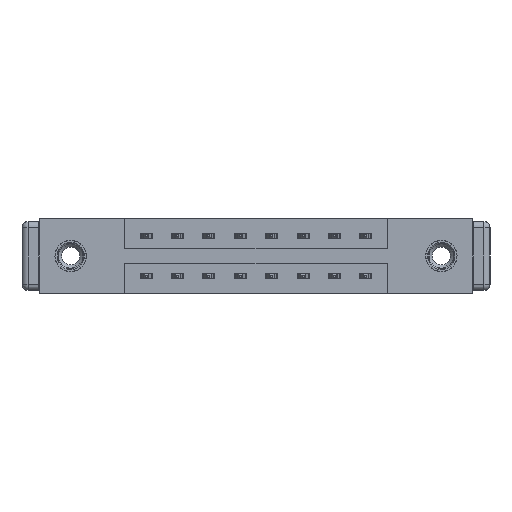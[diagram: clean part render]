
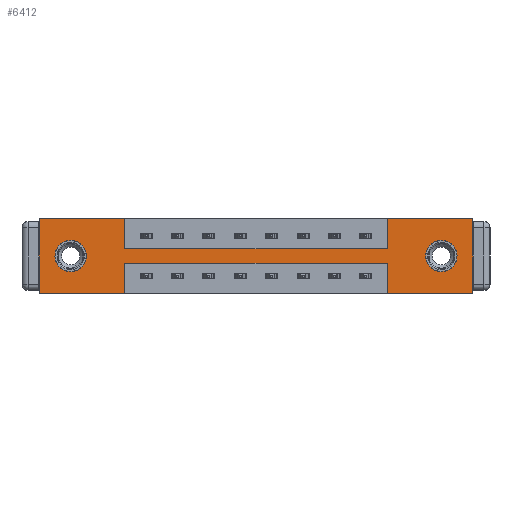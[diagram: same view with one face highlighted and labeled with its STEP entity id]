
A CAD part, front view. The second image highlights one B-rep face of the part: STEP entity #6412.
In plain terms, the highlighted planar face has unit normal (0, -1, 0).
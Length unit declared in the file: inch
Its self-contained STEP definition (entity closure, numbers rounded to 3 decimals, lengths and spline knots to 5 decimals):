
#91 = EDGE_CURVE ( 'NONE', #9414, #9587, #3976, .T. ) ;
#135 = FACE_BOUND ( 'NONE', #7141, .T. ) ;
#146 = VECTOR ( 'NONE', #11348, 39.37008 ) ;
#252 = DIRECTION ( 'NONE',  ( 0., 0., 1. ) ) ;
#331 = ORIENTED_EDGE ( 'NONE', *, *, #1827, .F. ) ;
#419 = DIRECTION ( 'NONE',  ( 0., 1., 0. ) ) ;
#629 = EDGE_CURVE ( 'NONE', #3409, #6597, #10270, .T. ) ;
#816 = ORIENTED_EDGE ( 'NONE', *, *, #9518, .F. ) ;
#857 = CARTESIAN_POINT ( 'NONE',  ( 1.729, 0., -0.15 ) ) ;
#905 = DIRECTION ( 'NONE',  ( 0., 0., -1. ) ) ;
#1058 = VECTOR ( 'NONE', #7113, 39.37008 ) ;
#1096 = CARTESIAN_POINT ( 'NONE',  ( 1.729, 0., -0.22 ) ) ;
#1280 = EDGE_CURVE ( 'NONE', #11914, #5512, #7104, .T. ) ;
#1364 = EDGE_CURVE ( 'NONE', #4600, #7504, #4291, .T. ) ;
#1548 = VECTOR ( 'NONE', #5077, 39.37008 ) ;
#1812 = DIRECTION ( 'NONE',  ( 0., 0., -1. ) ) ;
#1827 = EDGE_CURVE ( 'NONE', #2505, #9414, #9522, .T. ) ;
#1947 = CARTESIAN_POINT ( 'NONE',  ( 0.155, 0., -0.185 ) ) ;
#1994 = DIRECTION ( 'NONE',  ( 0., 0., 1. ) ) ;
#2085 = VERTEX_POINT ( 'NONE', #6038 ) ;
#2135 = LINE ( 'NONE', #4898, #11414 ) ;
#2250 = CARTESIAN_POINT ( 'NONE',  ( 0.155, 0., -0.185 ) ) ;
#2505 = VERTEX_POINT ( 'NONE', #5970 ) ;
#2510 = AXIS2_PLACEMENT_3D ( 'NONE', #1947, #7296, #1994 ) ;
#2540 = ORIENTED_EDGE ( 'NONE', *, *, #8767, .F. ) ;
#2572 = VERTEX_POINT ( 'NONE', #2990 ) ;
#2706 = ORIENTED_EDGE ( 'NONE', *, *, #6896, .F. ) ;
#2822 = PLANE ( 'NONE',  #11782 ) ;
#2990 = CARTESIAN_POINT ( 'NONE',  ( 0.425, 0., -0.22 ) ) ;
#3109 = CARTESIAN_POINT ( 'NONE',  ( 0., 0., 0. ) ) ;
#3409 = VERTEX_POINT ( 'NONE', #11630 ) ;
#3414 = DIRECTION ( 'NONE',  ( 1., 0., 0. ) ) ;
#3439 = CARTESIAN_POINT ( 'NONE',  ( 1.999, 0., -0.185 ) ) ;
#3529 = CARTESIAN_POINT ( 'NONE',  ( 0.425, 0., -0.22 ) ) ;
#3572 = VERTEX_POINT ( 'NONE', #4734 ) ;
#3855 = CARTESIAN_POINT ( 'NONE',  ( 2.154, 0., 0. ) ) ;
#3901 = VECTOR ( 'NONE', #8862, 39.37008 ) ;
#3939 = VERTEX_POINT ( 'NONE', #12723 ) ;
#3976 = LINE ( 'NONE', #6619, #5304 ) ;
#4216 = LINE ( 'NONE', #3529, #12200 ) ;
#4291 = LINE ( 'NONE', #3109, #146 ) ;
#4347 = ORIENTED_EDGE ( 'NONE', *, *, #13234, .F. ) ;
#4410 = ORIENTED_EDGE ( 'NONE', *, *, #8797, .F. ) ;
#4600 = VERTEX_POINT ( 'NONE', #4785 ) ;
#4614 = DIRECTION ( 'NONE',  ( -1., 0., 0. ) ) ;
#4734 = CARTESIAN_POINT ( 'NONE',  ( 1.999, 0., -0.263 ) ) ;
#4779 = EDGE_CURVE ( 'NONE', #8773, #8527, #4991, .T. ) ;
#4784 = CARTESIAN_POINT ( 'NONE',  ( 0.425, 0., 0. ) ) ;
#4785 = CARTESIAN_POINT ( 'NONE',  ( 0., 0., 0. ) ) ;
#4898 = CARTESIAN_POINT ( 'NONE',  ( 0.425, 0., -0.37 ) ) ;
#4899 = LINE ( 'NONE', #6059, #1058 ) ;
#4991 = CIRCLE ( 'NONE', #2510, 0.078 ) ;
#5077 = DIRECTION ( 'NONE',  ( 1., 0., 0. ) ) ;
#5133 = CARTESIAN_POINT ( 'NONE',  ( 1.999, 0., -0.185 ) ) ;
#5273 = FACE_BOUND ( 'NONE', #13248, .T. ) ;
#5304 = VECTOR ( 'NONE', #8513, 39.37008 ) ;
#5512 = VERTEX_POINT ( 'NONE', #6915 ) ;
#5582 = CARTESIAN_POINT ( 'NONE',  ( 0., 0., 0. ) ) ;
#5689 = CARTESIAN_POINT ( 'NONE',  ( 0.425, 0., 0. ) ) ;
#5869 = CIRCLE ( 'NONE', #12159, 0.078 ) ;
#5970 = CARTESIAN_POINT ( 'NONE',  ( 2.154, 0., 0. ) ) ;
#6038 = CARTESIAN_POINT ( 'NONE',  ( 0.425, 0., -0.15 ) ) ;
#6059 = CARTESIAN_POINT ( 'NONE',  ( 0., 0., 0. ) ) ;
#6123 = CARTESIAN_POINT ( 'NONE',  ( 2.154, 0., -0.37 ) ) ;
#6124 = VECTOR ( 'NONE', #12165, 39.37008 ) ;
#6165 = CARTESIAN_POINT ( 'NONE',  ( 0.425, 0., -0.15 ) ) ;
#6405 = AXIS2_PLACEMENT_3D ( 'NONE', #5133, #8371, #8412 ) ;
#6412 = ADVANCED_FACE ( 'NONE', ( #135, #5273, #11950 ), #2822, .T. ) ;
#6597 = VERTEX_POINT ( 'NONE', #13278 ) ;
#6619 = CARTESIAN_POINT ( 'NONE',  ( 0., 0., -0.37 ) ) ;
#6689 = VECTOR ( 'NONE', #7586, 39.37008 ) ;
#6895 = EDGE_CURVE ( 'NONE', #8527, #8773, #7016, .T. ) ;
#6896 = EDGE_CURVE ( 'NONE', #5512, #2505, #10242, .T. ) ;
#6915 = CARTESIAN_POINT ( 'NONE',  ( 1.729, 0., 0. ) ) ;
#6943 = ORIENTED_EDGE ( 'NONE', *, *, #13256, .T. ) ;
#6947 = CARTESIAN_POINT ( 'NONE',  ( 0.155, 0., -0.263 ) ) ;
#7016 = CIRCLE ( 'NONE', #8831, 0.078 ) ;
#7033 = LINE ( 'NONE', #5689, #6689 ) ;
#7104 = LINE ( 'NONE', #11126, #6124 ) ;
#7113 = DIRECTION ( 'NONE',  ( 0., 0., 1. ) ) ;
#7141 = EDGE_LOOP ( 'NONE', ( #12300, #6943 ) ) ;
#7296 = DIRECTION ( 'NONE',  ( 0., 1., 0. ) ) ;
#7504 = VERTEX_POINT ( 'NONE', #4784 ) ;
#7586 = DIRECTION ( 'NONE',  ( 0., 0., -1. ) ) ;
#7851 = CARTESIAN_POINT ( 'NONE',  ( 0., 0., -0.37 ) ) ;
#7904 = EDGE_CURVE ( 'NONE', #3939, #3572, #10973, .T. ) ;
#7933 = DIRECTION ( 'NONE',  ( 0., 0., -1. ) ) ;
#8047 = DIRECTION ( 'NONE',  ( 0., 0., 1. ) ) ;
#8069 = ORIENTED_EDGE ( 'NONE', *, *, #1280, .F. ) ;
#8371 = DIRECTION ( 'NONE',  ( 0., 1., 0. ) ) ;
#8412 = DIRECTION ( 'NONE',  ( 0., 0., -1. ) ) ;
#8513 = DIRECTION ( 'NONE',  ( -1., 0., 0. ) ) ;
#8527 = VERTEX_POINT ( 'NONE', #11638 ) ;
#8681 = CARTESIAN_POINT ( 'NONE',  ( 1.729, 0., -0.37 ) ) ;
#8767 = EDGE_CURVE ( 'NONE', #9587, #9375, #9828, .T. ) ;
#8773 = VERTEX_POINT ( 'NONE', #6947 ) ;
#8797 = EDGE_CURVE ( 'NONE', #2085, #11914, #12739, .T. ) ;
#8831 = AXIS2_PLACEMENT_3D ( 'NONE', #2250, #12695, #252 ) ;
#8862 = DIRECTION ( 'NONE',  ( -1., 0., 0. ) ) ;
#8959 = VECTOR ( 'NONE', #3414, 39.37008 ) ;
#8990 = DIRECTION ( 'NONE',  ( 0., 0., -1. ) ) ;
#9068 = EDGE_LOOP ( 'NONE', ( #11491, #11958, #2540, #9132, #331, #2706, #8069, #4410, #4347, #11704, #816, #9120 ) ) ;
#9120 = ORIENTED_EDGE ( 'NONE', *, *, #629, .F. ) ;
#9132 = ORIENTED_EDGE ( 'NONE', *, *, #91, .F. ) ;
#9375 = VERTEX_POINT ( 'NONE', #1096 ) ;
#9414 = VERTEX_POINT ( 'NONE', #6123 ) ;
#9518 = EDGE_CURVE ( 'NONE', #6597, #4600, #4899, .T. ) ;
#9522 = LINE ( 'NONE', #3855, #12590 ) ;
#9587 = VERTEX_POINT ( 'NONE', #13113 ) ;
#9828 = LINE ( 'NONE', #8681, #9996 ) ;
#9872 = EDGE_CURVE ( 'NONE', #2572, #3409, #2135, .T. ) ;
#9996 = VECTOR ( 'NONE', #8047, 39.37008 ) ;
#10242 = LINE ( 'NONE', #5582, #8959 ) ;
#10270 = LINE ( 'NONE', #7851, #3901 ) ;
#10973 = CIRCLE ( 'NONE', #6405, 0.078 ) ;
#11069 = CARTESIAN_POINT ( 'NONE',  ( 0., 0., -0.37 ) ) ;
#11108 = DIRECTION ( 'NONE',  ( 0., -1., 0. ) ) ;
#11126 = CARTESIAN_POINT ( 'NONE',  ( 1.729, 0., 0. ) ) ;
#11348 = DIRECTION ( 'NONE',  ( 1., 0., 0. ) ) ;
#11414 = VECTOR ( 'NONE', #905, 39.37008 ) ;
#11491 = ORIENTED_EDGE ( 'NONE', *, *, #9872, .F. ) ;
#11630 = CARTESIAN_POINT ( 'NONE',  ( 0.425, 0., -0.37 ) ) ;
#11638 = CARTESIAN_POINT ( 'NONE',  ( 0.155, 0., -0.107 ) ) ;
#11704 = ORIENTED_EDGE ( 'NONE', *, *, #1364, .F. ) ;
#11782 = AXIS2_PLACEMENT_3D ( 'NONE', #11069, #11108, #8990 ) ;
#11914 = VERTEX_POINT ( 'NONE', #857 ) ;
#11950 = FACE_OUTER_BOUND ( 'NONE', #9068, .T. ) ;
#11958 = ORIENTED_EDGE ( 'NONE', *, *, #13231, .F. ) ;
#12159 = AXIS2_PLACEMENT_3D ( 'NONE', #3439, #419, #7933 ) ;
#12165 = DIRECTION ( 'NONE',  ( 0., 0., 1. ) ) ;
#12200 = VECTOR ( 'NONE', #4614, 39.37008 ) ;
#12300 = ORIENTED_EDGE ( 'NONE', *, *, #7904, .T. ) ;
#12590 = VECTOR ( 'NONE', #1812, 39.37008 ) ;
#12695 = DIRECTION ( 'NONE',  ( 0., 1., 0. ) ) ;
#12723 = CARTESIAN_POINT ( 'NONE',  ( 1.999, 0., -0.107 ) ) ;
#12739 = LINE ( 'NONE', #6165, #1548 ) ;
#12820 = ORIENTED_EDGE ( 'NONE', *, *, #4779, .T. ) ;
#13113 = CARTESIAN_POINT ( 'NONE',  ( 1.729, 0., -0.37 ) ) ;
#13165 = ORIENTED_EDGE ( 'NONE', *, *, #6895, .T. ) ;
#13231 = EDGE_CURVE ( 'NONE', #9375, #2572, #4216, .T. ) ;
#13234 = EDGE_CURVE ( 'NONE', #7504, #2085, #7033, .T. ) ;
#13248 = EDGE_LOOP ( 'NONE', ( #13165, #12820 ) ) ;
#13256 = EDGE_CURVE ( 'NONE', #3572, #3939, #5869, .T. ) ;
#13278 = CARTESIAN_POINT ( 'NONE',  ( 0., 0., -0.37 ) ) ;
